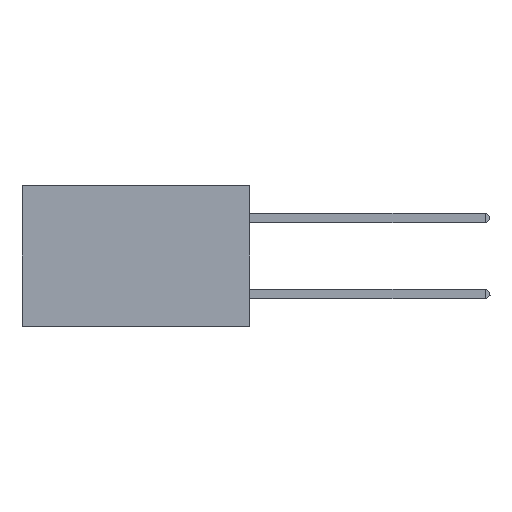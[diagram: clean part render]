
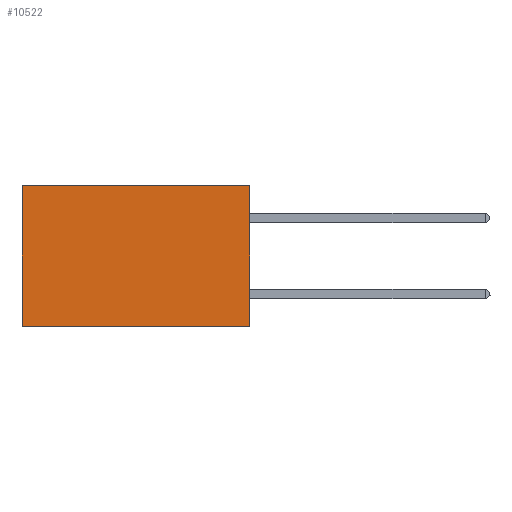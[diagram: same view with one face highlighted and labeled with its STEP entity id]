
A CAD part, left-side view. The second image highlights one B-rep face of the part: STEP entity #10522.
In plain terms, the highlighted planar face has unit normal (-1, 0, 0).
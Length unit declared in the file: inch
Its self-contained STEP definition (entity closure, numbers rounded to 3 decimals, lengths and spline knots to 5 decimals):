
#307 = VERTEX_POINT ( 'NONE', #9916 ) ;
#652 = EDGE_CURVE ( 'NONE', #11366, #307, #11340, .T. ) ;
#790 = VECTOR ( 'NONE', #5725, 39.37008 ) ;
#1089 = VECTOR ( 'NONE', #6434, 39.37008 ) ;
#1220 = CARTESIAN_POINT ( 'NONE',  ( 0.2875, 0., 0. ) ) ;
#1300 = CARTESIAN_POINT ( 'NONE',  ( 0.2875, 0., -0.37 ) ) ;
#2358 = CARTESIAN_POINT ( 'NONE',  ( 0.2875, 0., 0. ) ) ;
#2497 = EDGE_CURVE ( 'NONE', #8425, #11366, #9794, .T. ) ;
#3526 = AXIS2_PLACEMENT_3D ( 'NONE', #4194, #11447, #5298 ) ;
#3870 = VERTEX_POINT ( 'NONE', #13012 ) ;
#4194 = CARTESIAN_POINT ( 'NONE',  ( 0.2875, 0., 0. ) ) ;
#4214 = LINE ( 'NONE', #2358, #790 ) ;
#5298 = DIRECTION ( 'NONE',  ( 0., 0., -1. ) ) ;
#5681 = CARTESIAN_POINT ( 'NONE',  ( 0.2875, 0.6, 0. ) ) ;
#5725 = DIRECTION ( 'NONE',  ( 0., 1., 0. ) ) ;
#5892 = VECTOR ( 'NONE', #7515, 39.37008 ) ;
#6434 = DIRECTION ( 'NONE',  ( 0., 0., -1. ) ) ;
#6789 = DIRECTION ( 'NONE',  ( 0., 0., -1. ) ) ;
#7128 = EDGE_CURVE ( 'NONE', #3870, #307, #7768, .T. ) ;
#7515 = DIRECTION ( 'NONE',  ( 0., 1., 0. ) ) ;
#7768 = LINE ( 'NONE', #5681, #12749 ) ;
#8425 = VERTEX_POINT ( 'NONE', #13747 ) ;
#9506 = PLANE ( 'NONE',  #3526 ) ;
#9794 = LINE ( 'NONE', #1220, #1089 ) ;
#9873 = CARTESIAN_POINT ( 'NONE',  ( 0.2875, 0., -0.37 ) ) ;
#9916 = CARTESIAN_POINT ( 'NONE',  ( 0.2875, 0.6, -0.37 ) ) ;
#10374 = ORIENTED_EDGE ( 'NONE', *, *, #11934, .T. ) ;
#10522 = ADVANCED_FACE ( 'NONE', ( #11093 ), #9506, .F. ) ;
#11093 = FACE_OUTER_BOUND ( 'NONE', #12903, .T. ) ;
#11340 = LINE ( 'NONE', #9873, #5892 ) ;
#11366 = VERTEX_POINT ( 'NONE', #1300 ) ;
#11447 = DIRECTION ( 'NONE',  ( 1., 0., 0. ) ) ;
#11758 = ORIENTED_EDGE ( 'NONE', *, *, #2497, .F. ) ;
#11934 = EDGE_CURVE ( 'NONE', #8425, #3870, #4214, .T. ) ;
#12087 = ORIENTED_EDGE ( 'NONE', *, *, #652, .F. ) ;
#12749 = VECTOR ( 'NONE', #6789, 39.37008 ) ;
#12876 = ORIENTED_EDGE ( 'NONE', *, *, #7128, .T. ) ;
#12903 = EDGE_LOOP ( 'NONE', ( #12876, #12087, #11758, #10374 ) ) ;
#13012 = CARTESIAN_POINT ( 'NONE',  ( 0.2875, 0.6, 0. ) ) ;
#13747 = CARTESIAN_POINT ( 'NONE',  ( 0.2875, 0., 0. ) ) ;
